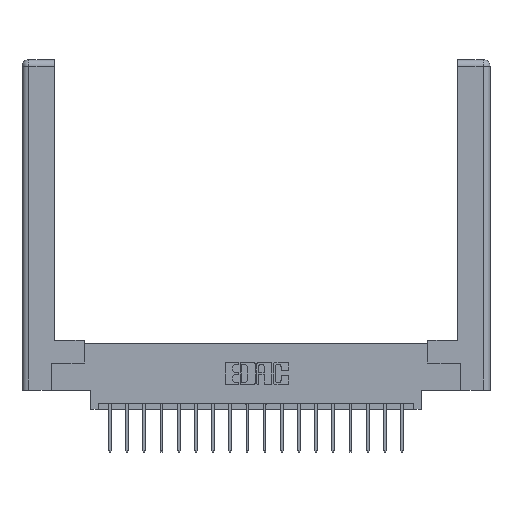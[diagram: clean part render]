
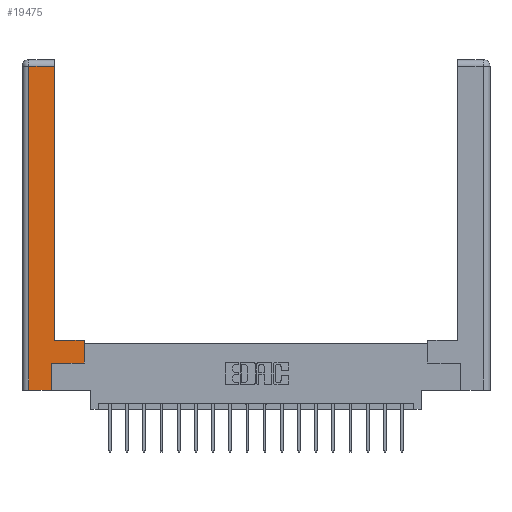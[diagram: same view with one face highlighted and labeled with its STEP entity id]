
A CAD part, top view. The second image highlights one B-rep face of the part: STEP entity #19475.
In plain terms, the highlighted planar face has unit normal (0, 0, 1).
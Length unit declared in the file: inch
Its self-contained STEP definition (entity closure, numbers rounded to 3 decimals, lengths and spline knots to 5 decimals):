
#355 = PLANE ( 'NONE',  #1536 ) ;
#739 = DIRECTION ( 'NONE',  ( 0., 1., 0. ) ) ;
#1536 = AXIS2_PLACEMENT_3D ( 'NONE', #17343, #8151, #1918 ) ;
#1598 = VECTOR ( 'NONE', #15137, 39.37008 ) ;
#1623 = CARTESIAN_POINT ( 'NONE',  ( 0.265, 0., 0. ) ) ;
#1675 = CARTESIAN_POINT ( 'NONE',  ( 0.295, 0.45, 0. ) ) ;
#1863 = EDGE_CURVE ( 'NONE', #11850, #16141, #5811, .T. ) ;
#1918 = DIRECTION ( 'NONE',  ( -1., 0., 0. ) ) ;
#2008 = VECTOR ( 'NONE', #12481, 39.37008 ) ;
#2120 = CARTESIAN_POINT ( 'NONE',  ( 0.565, 0.245, 0. ) ) ;
#2906 = CARTESIAN_POINT ( 'NONE',  ( 0.295, 0.45, 0. ) ) ;
#2916 = DIRECTION ( 'NONE',  ( 0., 1., 0. ) ) ;
#3109 = CARTESIAN_POINT ( 'NONE',  ( 0.295, 3., 0. ) ) ;
#3164 = LINE ( 'NONE', #10649, #11295 ) ;
#3416 = EDGE_CURVE ( 'NONE', #12469, #11850, #18984, .T. ) ;
#3638 = ORIENTED_EDGE ( 'NONE', *, *, #16832, .T. ) ;
#4457 = CARTESIAN_POINT ( 'NONE',  ( 0.565, 0.45, 0. ) ) ;
#4669 = ORIENTED_EDGE ( 'NONE', *, *, #15995, .T. ) ;
#4736 = ORIENTED_EDGE ( 'NONE', *, *, #18475, .T. ) ;
#4799 = CARTESIAN_POINT ( 'NONE',  ( 0.0615, 2.94, 0. ) ) ;
#4802 = EDGE_CURVE ( 'NONE', #4991, #11474, #3164, .T. ) ;
#4991 = VERTEX_POINT ( 'NONE', #14072 ) ;
#5811 = LINE ( 'NONE', #8811, #9877 ) ;
#6100 = ORIENTED_EDGE ( 'NONE', *, *, #16764, .T. ) ;
#6210 = CARTESIAN_POINT ( 'NONE',  ( 0.265, 0., 0. ) ) ;
#6729 = CARTESIAN_POINT ( 'NONE',  ( 0.0615, 0., 0. ) ) ;
#7131 = LINE ( 'NONE', #2906, #1598 ) ;
#7330 = VERTEX_POINT ( 'NONE', #16426 ) ;
#8151 = DIRECTION ( 'NONE',  ( 0., 0., -1. ) ) ;
#8811 = CARTESIAN_POINT ( 'NONE',  ( 0.0615, 0., 0. ) ) ;
#9393 = VERTEX_POINT ( 'NONE', #1675 ) ;
#9535 = VECTOR ( 'NONE', #14501, 39.37008 ) ;
#9680 = LINE ( 'NONE', #6210, #2008 ) ;
#9877 = VECTOR ( 'NONE', #13587, 39.37008 ) ;
#9951 = LINE ( 'NONE', #11542, #13053 ) ;
#10649 = CARTESIAN_POINT ( 'NONE',  ( 0.565, 0.45, 0. ) ) ;
#11295 = VECTOR ( 'NONE', #13982, 39.37008 ) ;
#11474 = VERTEX_POINT ( 'NONE', #4457 ) ;
#11542 = CARTESIAN_POINT ( 'NONE',  ( 0.265, 0.245, 0. ) ) ;
#11730 = CARTESIAN_POINT ( 'NONE',  ( 0.295, 2.94, 0. ) ) ;
#11850 = VERTEX_POINT ( 'NONE', #4799 ) ;
#11942 = CARTESIAN_POINT ( 'NONE',  ( 0.0615, 2.94, 0. ) ) ;
#12469 = VERTEX_POINT ( 'NONE', #11730 ) ;
#12481 = DIRECTION ( 'NONE',  ( 1., 0., 0. ) ) ;
#12864 = ORIENTED_EDGE ( 'NONE', *, *, #3416, .T. ) ;
#13053 = VECTOR ( 'NONE', #739, 39.37008 ) ;
#13525 = ORIENTED_EDGE ( 'NONE', *, *, #14713, .T. ) ;
#13587 = DIRECTION ( 'NONE',  ( 0., -1., 0. ) ) ;
#13982 = DIRECTION ( 'NONE',  ( 0., 1., 0. ) ) ;
#14072 = CARTESIAN_POINT ( 'NONE',  ( 0.565, 0.245, 0. ) ) ;
#14501 = DIRECTION ( 'NONE',  ( 1., 0., 0. ) ) ;
#14681 = ORIENTED_EDGE ( 'NONE', *, *, #1863, .T. ) ;
#14710 = ORIENTED_EDGE ( 'NONE', *, *, #4802, .T. ) ;
#14713 = EDGE_CURVE ( 'NONE', #19604, #7330, #9951, .T. ) ;
#14775 = VECTOR ( 'NONE', #2916, 39.37008 ) ;
#15137 = DIRECTION ( 'NONE',  ( -1., 0., 0. ) ) ;
#15995 = EDGE_CURVE ( 'NONE', #7330, #4991, #18180, .T. ) ;
#16141 = VERTEX_POINT ( 'NONE', #6729 ) ;
#16426 = CARTESIAN_POINT ( 'NONE',  ( 0.265, 0.245, 0. ) ) ;
#16764 = EDGE_CURVE ( 'NONE', #11474, #9393, #7131, .T. ) ;
#16832 = EDGE_CURVE ( 'NONE', #9393, #12469, #18878, .T. ) ;
#17284 = VECTOR ( 'NONE', #19659, 39.37008 ) ;
#17343 = CARTESIAN_POINT ( 'NONE',  ( 0., 0., 0. ) ) ;
#17735 = EDGE_LOOP ( 'NONE', ( #3638, #12864, #14681, #4736, #13525, #4669, #14710, #6100 ) ) ;
#17793 = FACE_OUTER_BOUND ( 'NONE', #17735, .T. ) ;
#18180 = LINE ( 'NONE', #2120, #9535 ) ;
#18475 = EDGE_CURVE ( 'NONE', #16141, #19604, #9680, .T. ) ;
#18878 = LINE ( 'NONE', #3109, #14775 ) ;
#18984 = LINE ( 'NONE', #11942, #17284 ) ;
#19475 = ADVANCED_FACE ( 'NONE', ( #17793 ), #355, .F. ) ;
#19604 = VERTEX_POINT ( 'NONE', #1623 ) ;
#19659 = DIRECTION ( 'NONE',  ( -1., 0., 0. ) ) ;
